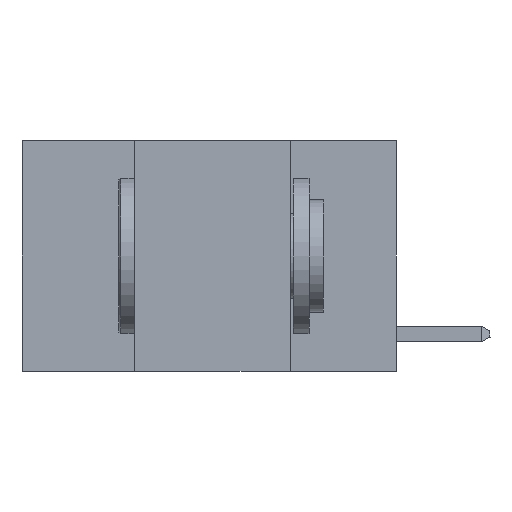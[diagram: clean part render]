
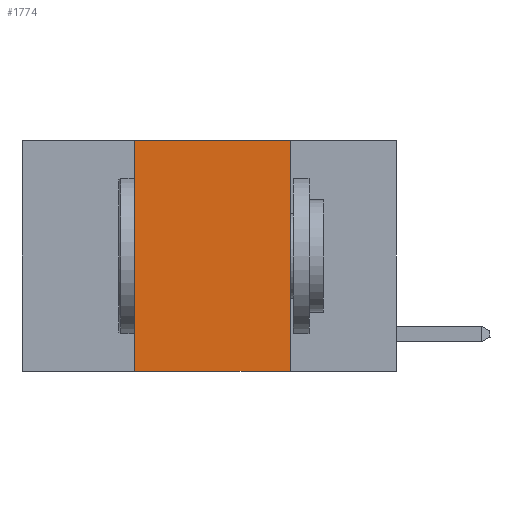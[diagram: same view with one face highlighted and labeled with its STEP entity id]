
A CAD part, left-side view. The second image highlights one B-rep face of the part: STEP entity #1774.
In plain terms, the highlighted planar face has unit normal (-1, 0, 0).
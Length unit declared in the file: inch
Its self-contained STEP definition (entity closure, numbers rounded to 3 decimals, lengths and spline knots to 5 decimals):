
#194 = CARTESIAN_POINT ( 'NONE',  ( 0., 0.6, -0.37 ) ) ;
#836 = DIRECTION ( 'NONE',  ( 0., 0., 1. ) ) ;
#930 = EDGE_CURVE ( 'NONE', #9275, #7350, #19821, .T. ) ;
#1159 = ORIENTED_EDGE ( 'NONE', *, *, #10772, .F. ) ;
#1182 = EDGE_CURVE ( 'NONE', #7350, #15040, #7805, .T. ) ;
#1774 = ADVANCED_FACE ( 'NONE', ( #9720 ), #19963, .F. ) ;
#2286 = VERTEX_POINT ( 'NONE', #17910 ) ;
#2615 = ORIENTED_EDGE ( 'NONE', *, *, #5569, .T. ) ;
#2951 = DIRECTION ( 'NONE',  ( 0., -1., 0. ) ) ;
#4440 = DIRECTION ( 'NONE',  ( 0., 0., -1. ) ) ;
#4832 = VECTOR ( 'NONE', #836, 39.37008 ) ;
#5569 = EDGE_CURVE ( 'NONE', #2286, #15040, #6033, .T. ) ;
#6033 = LINE ( 'NONE', #194, #18287 ) ;
#6166 = CARTESIAN_POINT ( 'NONE',  ( 0., 0.17, 0. ) ) ;
#7125 = CARTESIAN_POINT ( 'NONE',  ( 0., 0.42, 0. ) ) ;
#7350 = VERTEX_POINT ( 'NONE', #11145 ) ;
#7805 = LINE ( 'NONE', #6166, #10473 ) ;
#9275 = VERTEX_POINT ( 'NONE', #15921 ) ;
#9539 = CARTESIAN_POINT ( 'NONE',  ( 0., 0.17, -0.37 ) ) ;
#9617 = DIRECTION ( 'NONE',  ( 0., -1., 0. ) ) ;
#9720 = FACE_OUTER_BOUND ( 'NONE', #15182, .T. ) ;
#10473 = VECTOR ( 'NONE', #10509, 39.37008 ) ;
#10509 = DIRECTION ( 'NONE',  ( 0., 0., -1. ) ) ;
#10772 = EDGE_CURVE ( 'NONE', #2286, #9275, #17152, .T. ) ;
#11145 = CARTESIAN_POINT ( 'NONE',  ( 0., 0.17, 0. ) ) ;
#12850 = CARTESIAN_POINT ( 'NONE',  ( 0., 0.6, 0. ) ) ;
#14352 = ORIENTED_EDGE ( 'NONE', *, *, #1182, .F. ) ;
#15040 = VERTEX_POINT ( 'NONE', #9539 ) ;
#15182 = EDGE_LOOP ( 'NONE', ( #14352, #19822, #1159, #2615 ) ) ;
#15757 = VECTOR ( 'NONE', #2951, 39.37008 ) ;
#15921 = CARTESIAN_POINT ( 'NONE',  ( 0., 0.42, 0. ) ) ;
#16126 = AXIS2_PLACEMENT_3D ( 'NONE', #18440, #19406, #4440 ) ;
#17152 = LINE ( 'NONE', #7125, #4832 ) ;
#17910 = CARTESIAN_POINT ( 'NONE',  ( 0., 0.42, -0.37 ) ) ;
#18287 = VECTOR ( 'NONE', #9617, 39.37008 ) ;
#18440 = CARTESIAN_POINT ( 'NONE',  ( 0., 0.6, 0. ) ) ;
#19406 = DIRECTION ( 'NONE',  ( 1., 0., 0. ) ) ;
#19821 = LINE ( 'NONE', #12850, #15757 ) ;
#19822 = ORIENTED_EDGE ( 'NONE', *, *, #930, .F. ) ;
#19963 = PLANE ( 'NONE',  #16126 ) ;
